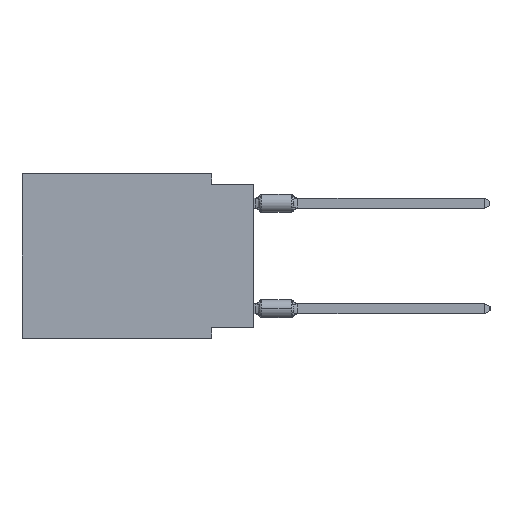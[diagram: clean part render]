
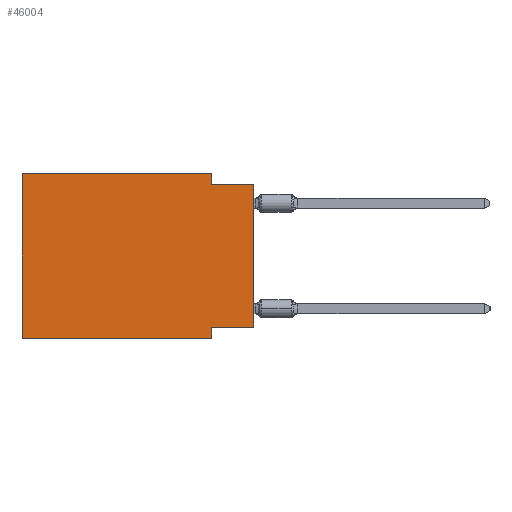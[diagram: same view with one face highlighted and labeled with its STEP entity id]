
A CAD part, left-side view. The second image highlights one B-rep face of the part: STEP entity #46004.
In plain terms, the highlighted planar face has unit normal (-1, 0, 0).
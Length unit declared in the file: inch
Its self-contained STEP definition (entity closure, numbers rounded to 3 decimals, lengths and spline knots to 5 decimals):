
#1530 = VECTOR ( 'NONE', #15314, 39.37008 ) ;
#1866 = CARTESIAN_POINT ( 'NONE',  ( 0., 0., -0.365 ) ) ;
#1868 = ORIENTED_EDGE ( 'NONE', *, *, #14998, .F. ) ;
#2876 = ORIENTED_EDGE ( 'NONE', *, *, #9544, .T. ) ;
#4239 = CARTESIAN_POINT ( 'NONE',  ( 0., 0.1, 0. ) ) ;
#5501 = EDGE_CURVE ( 'NONE', #59903, #7930, #24935, .T. ) ;
#7293 = EDGE_CURVE ( 'NONE', #59903, #14405, #15262, .T. ) ;
#7930 = VERTEX_POINT ( 'NONE', #44501 ) ;
#9059 = VERTEX_POINT ( 'NONE', #51049 ) ;
#9509 = VERTEX_POINT ( 'NONE', #52294 ) ;
#9544 = EDGE_CURVE ( 'NONE', #9509, #9059, #20797, .T. ) ;
#10987 = ORIENTED_EDGE ( 'NONE', *, *, #18463, .F. ) ;
#11804 = VERTEX_POINT ( 'NONE', #47243 ) ;
#12732 = ORIENTED_EDGE ( 'NONE', *, *, #7293, .T. ) ;
#13629 = DIRECTION ( 'NONE',  ( 0., -1., 0. ) ) ;
#14405 = VERTEX_POINT ( 'NONE', #45697 ) ;
#14998 = EDGE_CURVE ( 'NONE', #7930, #9059, #33730, .T. ) ;
#15262 = LINE ( 'NONE', #60150, #54689 ) ;
#15314 = DIRECTION ( 'NONE',  ( 0., 0., -1. ) ) ;
#18119 = CARTESIAN_POINT ( 'NONE',  ( 0., 0.55, 0. ) ) ;
#18369 = VECTOR ( 'NONE', #18783, 39.37008 ) ;
#18463 = EDGE_CURVE ( 'NONE', #21756, #32215, #35077, .T. ) ;
#18722 = ORIENTED_EDGE ( 'NONE', *, *, #5501, .F. ) ;
#18772 = FACE_OUTER_BOUND ( 'NONE', #65002, .T. ) ;
#18783 = DIRECTION ( 'NONE',  ( 0., 0., 1. ) ) ;
#20797 = LINE ( 'NONE', #30832, #38844 ) ;
#21756 = VERTEX_POINT ( 'NONE', #27691 ) ;
#22809 = LINE ( 'NONE', #18119, #18369 ) ;
#23170 = VECTOR ( 'NONE', #54520, 39.37008 ) ;
#24935 = LINE ( 'NONE', #45398, #30078 ) ;
#26458 = DIRECTION ( 'NONE',  ( 0., -1., 0. ) ) ;
#27408 = EDGE_CURVE ( 'NONE', #9509, #11804, #22809, .T. ) ;
#27691 = CARTESIAN_POINT ( 'NONE',  ( 0., 0.1, 0. ) ) ;
#28844 = ORIENTED_EDGE ( 'NONE', *, *, #58465, .F. ) ;
#29964 = CARTESIAN_POINT ( 'NONE',  ( 0., 0., -0.025 ) ) ;
#30078 = VECTOR ( 'NONE', #31617, 39.37008 ) ;
#30832 = CARTESIAN_POINT ( 'NONE',  ( 0., 0.55, -0.39 ) ) ;
#31617 = DIRECTION ( 'NONE',  ( 0., 1., 0. ) ) ;
#32215 = VERTEX_POINT ( 'NONE', #47730 ) ;
#33730 = LINE ( 'NONE', #64548, #23170 ) ;
#35077 = LINE ( 'NONE', #4239, #1530 ) ;
#36168 = PLANE ( 'NONE',  #55175 ) ;
#38844 = VECTOR ( 'NONE', #26458, 39.37008 ) ;
#39081 = LINE ( 'NONE', #59513, #59740 ) ;
#39373 = VECTOR ( 'NONE', #39715, 39.37008 ) ;
#39715 = DIRECTION ( 'NONE',  ( 0., -1., 0. ) ) ;
#40531 = DIRECTION ( 'NONE',  ( 0., 0., -1. ) ) ;
#43767 = LINE ( 'NONE', #29964, #39373 ) ;
#44501 = CARTESIAN_POINT ( 'NONE',  ( 0., 0.1, -0.365 ) ) ;
#45398 = CARTESIAN_POINT ( 'NONE',  ( 0., 0., -0.365 ) ) ;
#45697 = CARTESIAN_POINT ( 'NONE',  ( 0., 0., -0.025 ) ) ;
#46004 = ADVANCED_FACE ( 'NONE', ( #18772 ), #36168, .F. ) ;
#47243 = CARTESIAN_POINT ( 'NONE',  ( 0., 0.55, 0. ) ) ;
#47730 = CARTESIAN_POINT ( 'NONE',  ( 0., 0.1, -0.025 ) ) ;
#50110 = DIRECTION ( 'NONE',  ( 0., 0., 1. ) ) ;
#51049 = CARTESIAN_POINT ( 'NONE',  ( 0., 0.1, -0.39 ) ) ;
#51606 = ORIENTED_EDGE ( 'NONE', *, *, #57687, .F. ) ;
#52294 = CARTESIAN_POINT ( 'NONE',  ( 0., 0.55, -0.39 ) ) ;
#54520 = DIRECTION ( 'NONE',  ( 0., 0., -1. ) ) ;
#54689 = VECTOR ( 'NONE', #50110, 39.37008 ) ;
#55175 = AXIS2_PLACEMENT_3D ( 'NONE', #61626, #60301, #40531 ) ;
#57687 = EDGE_CURVE ( 'NONE', #32215, #14405, #43767, .T. ) ;
#58465 = EDGE_CURVE ( 'NONE', #11804, #21756, #39081, .T. ) ;
#59513 = CARTESIAN_POINT ( 'NONE',  ( 0., 0.55, 0. ) ) ;
#59740 = VECTOR ( 'NONE', #13629, 39.37008 ) ;
#59903 = VERTEX_POINT ( 'NONE', #1866 ) ;
#60150 = CARTESIAN_POINT ( 'NONE',  ( 0., 0., 0. ) ) ;
#60301 = DIRECTION ( 'NONE',  ( 1., 0., 0. ) ) ;
#61626 = CARTESIAN_POINT ( 'NONE',  ( 0., 0.55, 0. ) ) ;
#62488 = ORIENTED_EDGE ( 'NONE', *, *, #27408, .F. ) ;
#64548 = CARTESIAN_POINT ( 'NONE',  ( 0., 0.1, -0.39 ) ) ;
#65002 = EDGE_LOOP ( 'NONE', ( #12732, #51606, #10987, #28844, #62488, #2876, #1868, #18722 ) ) ;
